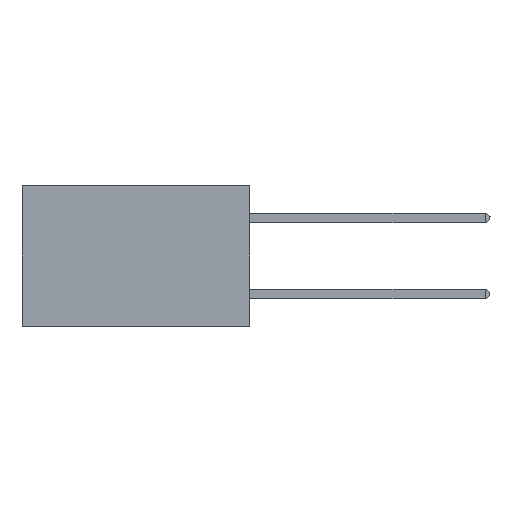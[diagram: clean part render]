
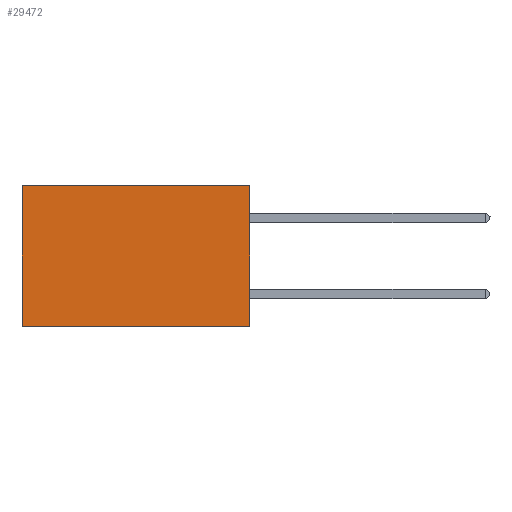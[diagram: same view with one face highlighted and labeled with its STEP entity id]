
A CAD part, left-side view. The second image highlights one B-rep face of the part: STEP entity #29472.
In plain terms, the highlighted planar face has unit normal (-1, 0, 0).
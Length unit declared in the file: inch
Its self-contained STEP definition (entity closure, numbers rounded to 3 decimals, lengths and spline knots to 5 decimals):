
#913 = ORIENTED_EDGE ( 'NONE', *, *, #3540, .F. ) ;
#1665 = PLANE ( 'NONE',  #5537 ) ;
#2360 = CARTESIAN_POINT ( 'NONE',  ( 0.2875, 0.6, -0.37 ) ) ;
#3023 = LINE ( 'NONE', #9324, #18543 ) ;
#3540 = EDGE_CURVE ( 'NONE', #36528, #38181, #20285, .T. ) ;
#3780 = VECTOR ( 'NONE', #29239, 39.37008 ) ;
#4609 = EDGE_LOOP ( 'NONE', ( #6337, #913, #16226, #33920 ) ) ;
#4789 = DIRECTION ( 'NONE',  ( 1., 0., 0. ) ) ;
#5537 = AXIS2_PLACEMENT_3D ( 'NONE', #23366, #4789, #26467 ) ;
#5986 = VERTEX_POINT ( 'NONE', #29478 ) ;
#6337 = ORIENTED_EDGE ( 'NONE', *, *, #37157, .T. ) ;
#8591 = DIRECTION ( 'NONE',  ( 0., 0., -1. ) ) ;
#9324 = CARTESIAN_POINT ( 'NONE',  ( 0.2875, 0., 0. ) ) ;
#13792 = CARTESIAN_POINT ( 'NONE',  ( 0.2875, 0., -0.37 ) ) ;
#16226 = ORIENTED_EDGE ( 'NONE', *, *, #23533, .F. ) ;
#18105 = CARTESIAN_POINT ( 'NONE',  ( 0.2875, 0., -0.37 ) ) ;
#18543 = VECTOR ( 'NONE', #37006, 39.37008 ) ;
#19011 = EDGE_CURVE ( 'NONE', #5986, #35479, #3023, .T. ) ;
#19505 = DIRECTION ( 'NONE',  ( 0., 0., -1. ) ) ;
#20285 = LINE ( 'NONE', #13792, #3780 ) ;
#23156 = LINE ( 'NONE', #24027, #31321 ) ;
#23366 = CARTESIAN_POINT ( 'NONE',  ( 0.2875, 0., 0. ) ) ;
#23533 = EDGE_CURVE ( 'NONE', #5986, #36528, #26151, .T. ) ;
#24027 = CARTESIAN_POINT ( 'NONE',  ( 0.2875, 0.6, 0. ) ) ;
#26151 = LINE ( 'NONE', #37833, #35242 ) ;
#26467 = DIRECTION ( 'NONE',  ( 0., 0., -1. ) ) ;
#29239 = DIRECTION ( 'NONE',  ( 0., 1., 0. ) ) ;
#29472 = ADVANCED_FACE ( 'NONE', ( #35307 ), #1665, .F. ) ;
#29478 = CARTESIAN_POINT ( 'NONE',  ( 0.2875, 0., 0. ) ) ;
#31321 = VECTOR ( 'NONE', #8591, 39.37008 ) ;
#33920 = ORIENTED_EDGE ( 'NONE', *, *, #19011, .T. ) ;
#34981 = CARTESIAN_POINT ( 'NONE',  ( 0.2875, 0.6, 0. ) ) ;
#35242 = VECTOR ( 'NONE', #19505, 39.37008 ) ;
#35307 = FACE_OUTER_BOUND ( 'NONE', #4609, .T. ) ;
#35479 = VERTEX_POINT ( 'NONE', #34981 ) ;
#36528 = VERTEX_POINT ( 'NONE', #18105 ) ;
#37006 = DIRECTION ( 'NONE',  ( 0., 1., 0. ) ) ;
#37157 = EDGE_CURVE ( 'NONE', #35479, #38181, #23156, .T. ) ;
#37833 = CARTESIAN_POINT ( 'NONE',  ( 0.2875, 0., 0. ) ) ;
#38181 = VERTEX_POINT ( 'NONE', #2360 ) ;
